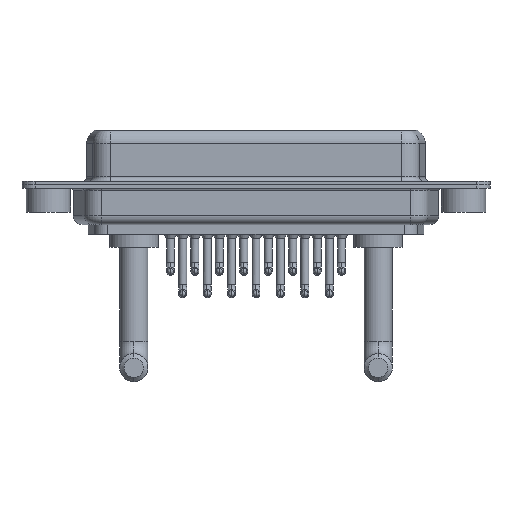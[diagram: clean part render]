
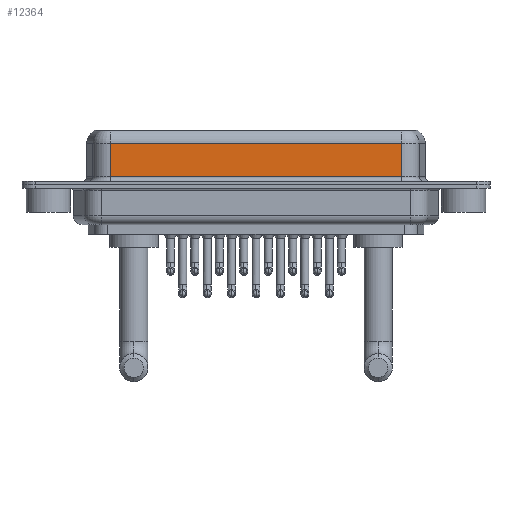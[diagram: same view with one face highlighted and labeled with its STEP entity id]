
A CAD part, front view. The second image highlights one B-rep face of the part: STEP entity #12364.
In plain terms, the highlighted planar face has unit normal (0, -1, 0).
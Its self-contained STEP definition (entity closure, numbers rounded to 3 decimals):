
#871 = CARTESIAN_POINT ( 'NONE',  ( 40.037, -3.95, 0.9 ) ) ;
#1912 = DIRECTION ( 'NONE',  ( 0., 1., 0. ) ) ;
#2084 = VECTOR ( 'NONE', #14736, 1000. ) ;
#2111 = CARTESIAN_POINT ( 'NONE',  ( 40.037, -3.95, 6.4 ) ) ;
#2283 = VECTOR ( 'NONE', #7296, 1000. ) ;
#2655 = CARTESIAN_POINT ( 'NONE',  ( 40.037, -3.95, 4.65 ) ) ;
#2727 = VERTEX_POINT ( 'NONE', #7877 ) ;
#2844 = EDGE_CURVE ( 'NONE', #6941, #2727, #8397, .T. ) ;
#3436 = ORIENTED_EDGE ( 'NONE', *, *, #17806, .T. ) ;
#3966 = EDGE_CURVE ( 'NONE', #6941, #19614, #10678, .T. ) ;
#5623 = CARTESIAN_POINT ( 'NONE',  ( 40.037, -3.95, 6.4 ) ) ;
#6941 = VERTEX_POINT ( 'NONE', #2655 ) ;
#7296 = DIRECTION ( 'NONE',  ( 1., 0., 0. ) ) ;
#7877 = CARTESIAN_POINT ( 'NONE',  ( 7.013, -3.95, 4.65 ) ) ;
#8042 = CARTESIAN_POINT ( 'NONE',  ( 40.037, -3.95, 0.9 ) ) ;
#8077 = ORIENTED_EDGE ( 'NONE', *, *, #16229, .T. ) ;
#8222 = PLANE ( 'NONE',  #9570 ) ;
#8337 = CARTESIAN_POINT ( 'NONE',  ( 7.013, -3.95, 6.4 ) ) ;
#8397 = LINE ( 'NONE', #14827, #2084 ) ;
#8425 = DIRECTION ( 'NONE',  ( 0., 0., 1. ) ) ;
#8529 = FACE_OUTER_BOUND ( 'NONE', #16480, .T. ) ;
#9570 = AXIS2_PLACEMENT_3D ( 'NONE', #2111, #1912, #8425 ) ;
#9881 = VECTOR ( 'NONE', #16457, 1000. ) ;
#10124 = LINE ( 'NONE', #871, #2283 ) ;
#10678 = LINE ( 'NONE', #5623, #15536 ) ;
#11296 = LINE ( 'NONE', #8337, #9881 ) ;
#12364 = ADVANCED_FACE ( 'NONE', ( #8529 ), #8222, .F. ) ;
#12537 = ORIENTED_EDGE ( 'NONE', *, *, #2844, .T. ) ;
#13491 = VERTEX_POINT ( 'NONE', #18888 ) ;
#14736 = DIRECTION ( 'NONE',  ( -1., 0., 0. ) ) ;
#14827 = CARTESIAN_POINT ( 'NONE',  ( 40.037, -3.95, 4.65 ) ) ;
#15419 = DIRECTION ( 'NONE',  ( 0., 0., -1. ) ) ;
#15536 = VECTOR ( 'NONE', #15419, 1000. ) ;
#16229 = EDGE_CURVE ( 'NONE', #13491, #19614, #10124, .T. ) ;
#16457 = DIRECTION ( 'NONE',  ( 0., 0., -1. ) ) ;
#16480 = EDGE_LOOP ( 'NONE', ( #16654, #12537, #3436, #8077 ) ) ;
#16654 = ORIENTED_EDGE ( 'NONE', *, *, #3966, .F. ) ;
#17806 = EDGE_CURVE ( 'NONE', #2727, #13491, #11296, .T. ) ;
#18888 = CARTESIAN_POINT ( 'NONE',  ( 7.013, -3.95, 0.9 ) ) ;
#19614 = VERTEX_POINT ( 'NONE', #8042 ) ;
